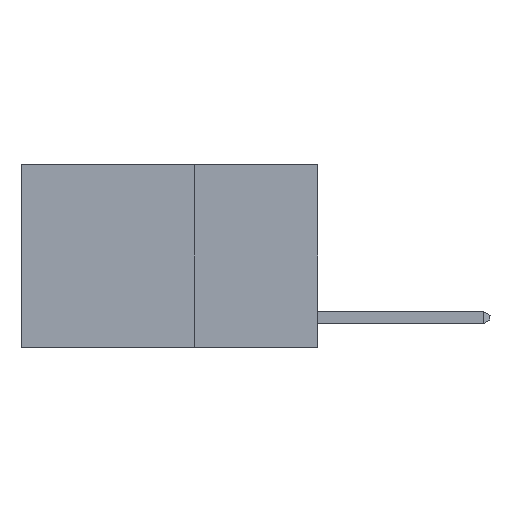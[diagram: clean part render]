
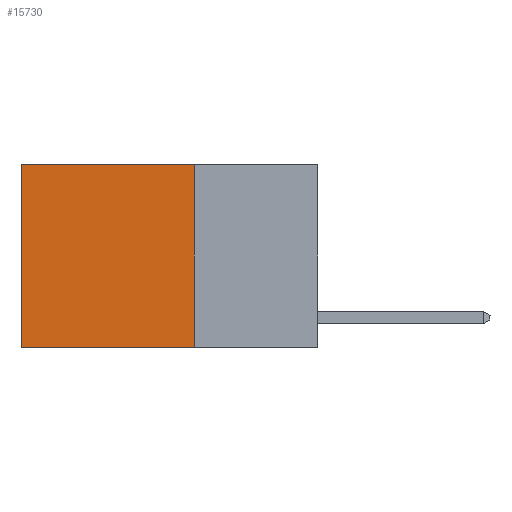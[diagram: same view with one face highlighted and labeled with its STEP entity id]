
A CAD part, left-side view. The second image highlights one B-rep face of the part: STEP entity #15730.
In plain terms, the highlighted planar face has unit normal (-1, 0, 0).
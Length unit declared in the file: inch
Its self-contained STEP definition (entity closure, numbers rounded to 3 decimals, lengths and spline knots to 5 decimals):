
#563 = PLANE ( 'NONE',  #1686 ) ;
#647 = ORIENTED_EDGE ( 'NONE', *, *, #4699, .F. ) ;
#684 = LINE ( 'NONE', #7624, #10740 ) ;
#762 = FACE_OUTER_BOUND ( 'NONE', #16981, .T. ) ;
#1309 = VECTOR ( 'NONE', #14801, 39.37008 ) ;
#1437 = DIRECTION ( 'NONE',  ( 0., 0., -1. ) ) ;
#1686 = AXIS2_PLACEMENT_3D ( 'NONE', #6800, #2405, #5119 ) ;
#2305 = EDGE_CURVE ( 'NONE', #14807, #15643, #11691, .T. ) ;
#2405 = DIRECTION ( 'NONE',  ( 1., 0., 0. ) ) ;
#3143 = EDGE_CURVE ( 'NONE', #3777, #15643, #8635, .T. ) ;
#3777 = VERTEX_POINT ( 'NONE', #13012 ) ;
#4699 = EDGE_CURVE ( 'NONE', #17471, #14807, #11483, .T. ) ;
#5119 = DIRECTION ( 'NONE',  ( 0., 0., -1. ) ) ;
#6800 = CARTESIAN_POINT ( 'NONE',  ( 0.2625, 0.25, 0. ) ) ;
#7624 = CARTESIAN_POINT ( 'NONE',  ( 0.2625, 0.25, 0. ) ) ;
#8209 = VECTOR ( 'NONE', #1437, 39.37008 ) ;
#8635 = LINE ( 'NONE', #18843, #8209 ) ;
#10740 = VECTOR ( 'NONE', #18566, 39.37008 ) ;
#11483 = LINE ( 'NONE', #15494, #13618 ) ;
#11691 = LINE ( 'NONE', #15965, #1309 ) ;
#13012 = CARTESIAN_POINT ( 'NONE',  ( 0.2625, 0.6, 0. ) ) ;
#13136 = DIRECTION ( 'NONE',  ( 0., 0., -1. ) ) ;
#13618 = VECTOR ( 'NONE', #13136, 39.37008 ) ;
#14001 = ORIENTED_EDGE ( 'NONE', *, *, #2305, .F. ) ;
#14801 = DIRECTION ( 'NONE',  ( 0., 1., 0. ) ) ;
#14807 = VERTEX_POINT ( 'NONE', #19222 ) ;
#15494 = CARTESIAN_POINT ( 'NONE',  ( 0.2625, 0.25, 0. ) ) ;
#15643 = VERTEX_POINT ( 'NONE', #16419 ) ;
#15730 = ADVANCED_FACE ( 'NONE', ( #762 ), #563, .F. ) ;
#15965 = CARTESIAN_POINT ( 'NONE',  ( 0.2625, 0.25, -0.37 ) ) ;
#16419 = CARTESIAN_POINT ( 'NONE',  ( 0.2625, 0.6, -0.37 ) ) ;
#16573 = CARTESIAN_POINT ( 'NONE',  ( 0.2625, 0.25, 0. ) ) ;
#16931 = ORIENTED_EDGE ( 'NONE', *, *, #3143, .T. ) ;
#16981 = EDGE_LOOP ( 'NONE', ( #16931, #14001, #647, #17050 ) ) ;
#17050 = ORIENTED_EDGE ( 'NONE', *, *, #17802, .T. ) ;
#17471 = VERTEX_POINT ( 'NONE', #16573 ) ;
#17802 = EDGE_CURVE ( 'NONE', #17471, #3777, #684, .T. ) ;
#18566 = DIRECTION ( 'NONE',  ( 0., 1., 0. ) ) ;
#18843 = CARTESIAN_POINT ( 'NONE',  ( 0.2625, 0.6, 0. ) ) ;
#19222 = CARTESIAN_POINT ( 'NONE',  ( 0.2625, 0.25, -0.37 ) ) ;
